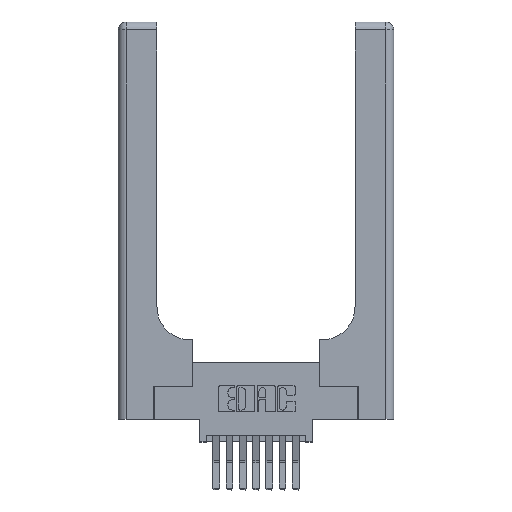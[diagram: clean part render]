
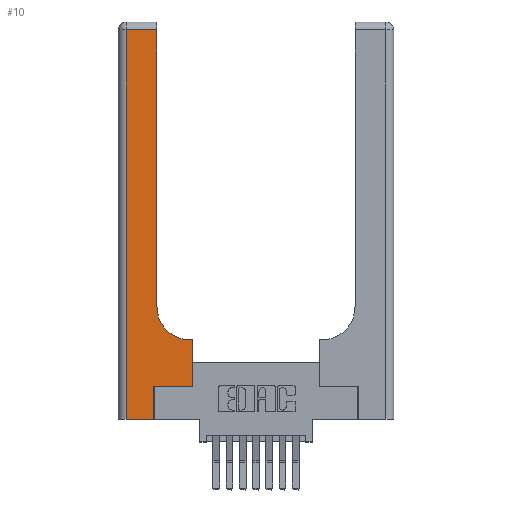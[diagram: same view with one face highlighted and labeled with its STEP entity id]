
A CAD part, top view. The second image highlights one B-rep face of the part: STEP entity #10.
In plain terms, the highlighted planar face has unit normal (0, 0, 1).
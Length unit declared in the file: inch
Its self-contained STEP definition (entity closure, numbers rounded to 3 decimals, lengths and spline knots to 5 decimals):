
#10 = ADVANCED_FACE ( 'NONE', ( #7738 ), #1130, .F. ) ;
#654 = LINE ( 'NONE', #7620, #6672 ) ;
#670 = CARTESIAN_POINT ( 'NONE',  ( 0.2915, 0.6, 0.37 ) ) ;
#739 = VECTOR ( 'NONE', #13479, 39.37008 ) ;
#786 = LINE ( 'NONE', #11193, #13255 ) ;
#826 = ORIENTED_EDGE ( 'NONE', *, *, #11435, .T. ) ;
#1130 = PLANE ( 'NONE',  #12716 ) ;
#1564 = ORIENTED_EDGE ( 'NONE', *, *, #3836, .T. ) ;
#1618 = LINE ( 'NONE', #4243, #4477 ) ;
#1707 = CARTESIAN_POINT ( 'NONE',  ( 0.5415, 0.85, 0.37 ) ) ;
#1835 = CARTESIAN_POINT ( 'NONE',  ( 0.06, 2.94, 0.37 ) ) ;
#2372 = ORIENTED_EDGE ( 'NONE', *, *, #14680, .T. ) ;
#2967 = DIRECTION ( 'NONE',  ( 1., 0., 0. ) ) ;
#3564 = VERTEX_POINT ( 'NONE', #5213 ) ;
#3594 = CARTESIAN_POINT ( 'NONE',  ( 0.2915, 3., 0.37 ) ) ;
#3836 = EDGE_CURVE ( 'NONE', #8129, #15580, #4797, .T. ) ;
#3838 = CARTESIAN_POINT ( 'NONE',  ( 0.06, 3., 0.37 ) ) ;
#4243 = CARTESIAN_POINT ( 'NONE',  ( 0.269, 0.25, 0.37 ) ) ;
#4425 = ORIENTED_EDGE ( 'NONE', *, *, #7631, .T. ) ;
#4477 = VECTOR ( 'NONE', #11522, 39.37008 ) ;
#4797 = LINE ( 'NONE', #6931, #7634 ) ;
#5213 = CARTESIAN_POINT ( 'NONE',  ( 0.2915, 2.94, 0.37 ) ) ;
#5412 = EDGE_CURVE ( 'NONE', #14479, #10782, #786, .T. ) ;
#5531 = VERTEX_POINT ( 'NONE', #1835 ) ;
#5629 = EDGE_LOOP ( 'NONE', ( #10140, #826, #4425, #10887, #1564, #14407, #8391, #11648, #2372 ) ) ;
#6672 = VECTOR ( 'NONE', #8851, 39.37008 ) ;
#6785 = EDGE_CURVE ( 'NONE', #8385, #3564, #14325, .T. ) ;
#6931 = CARTESIAN_POINT ( 'NONE',  ( 0.269, 0., 0.37 ) ) ;
#6965 = DIRECTION ( 'NONE',  ( 0., 0., -1. ) ) ;
#7145 = LINE ( 'NONE', #3838, #739 ) ;
#7150 = CARTESIAN_POINT ( 'NONE',  ( 0.06, 0., 0.37 ) ) ;
#7544 = DIRECTION ( 'NONE',  ( 0., 1., 0. ) ) ;
#7587 = VECTOR ( 'NONE', #14410, 39.37008 ) ;
#7620 = CARTESIAN_POINT ( 'NONE',  ( 0., 2.94, 0.37 ) ) ;
#7631 = EDGE_CURVE ( 'NONE', #5531, #14396, #7145, .T. ) ;
#7634 = VECTOR ( 'NONE', #11798, 39.37008 ) ;
#7738 = FACE_OUTER_BOUND ( 'NONE', #5629, .T. ) ;
#8129 = VERTEX_POINT ( 'NONE', #12398 ) ;
#8385 = VERTEX_POINT ( 'NONE', #11726 ) ;
#8391 = ORIENTED_EDGE ( 'NONE', *, *, #5412, .T. ) ;
#8716 = CIRCLE ( 'NONE', #13418, 0.25 ) ;
#8841 = DIRECTION ( 'NONE',  ( 0., 1., 0. ) ) ;
#8851 = DIRECTION ( 'NONE',  ( -1., 0., 0. ) ) ;
#9270 = VERTEX_POINT ( 'NONE', #13484 ) ;
#9622 = CARTESIAN_POINT ( 'NONE',  ( 0., 0., 0.37 ) ) ;
#10137 = EDGE_CURVE ( 'NONE', #15580, #14479, #1618, .T. ) ;
#10140 = ORIENTED_EDGE ( 'NONE', *, *, #6785, .T. ) ;
#10224 = DIRECTION ( 'NONE',  ( 0., 0., -1. ) ) ;
#10391 = DIRECTION ( 'NONE',  ( -1., 0., 0. ) ) ;
#10782 = VERTEX_POINT ( 'NONE', #11017 ) ;
#10857 = LINE ( 'NONE', #9622, #7587 ) ;
#10887 = ORIENTED_EDGE ( 'NONE', *, *, #13054, .T. ) ;
#11005 = DIRECTION ( 'NONE',  ( -1., 0., 0. ) ) ;
#11017 = CARTESIAN_POINT ( 'NONE',  ( 0.5585, 0.6, 0.37 ) ) ;
#11193 = CARTESIAN_POINT ( 'NONE',  ( 0.5585, 0.25, 0.37 ) ) ;
#11435 = EDGE_CURVE ( 'NONE', #3564, #5531, #654, .T. ) ;
#11522 = DIRECTION ( 'NONE',  ( 1., 0., 0. ) ) ;
#11648 = ORIENTED_EDGE ( 'NONE', *, *, #12719, .T. ) ;
#11726 = CARTESIAN_POINT ( 'NONE',  ( 0.2915, 0.85, 0.37 ) ) ;
#11798 = DIRECTION ( 'NONE',  ( 0., 1., 0. ) ) ;
#12170 = VECTOR ( 'NONE', #10391, 39.37008 ) ;
#12398 = CARTESIAN_POINT ( 'NONE',  ( 0.269, 0., 0.37 ) ) ;
#12716 = AXIS2_PLACEMENT_3D ( 'NONE', #14660, #6965, #11005 ) ;
#12719 = EDGE_CURVE ( 'NONE', #10782, #9270, #12910, .T. ) ;
#12910 = LINE ( 'NONE', #670, #12170 ) ;
#13054 = EDGE_CURVE ( 'NONE', #14396, #8129, #10857, .T. ) ;
#13255 = VECTOR ( 'NONE', #7544, 39.37008 ) ;
#13418 = AXIS2_PLACEMENT_3D ( 'NONE', #1707, #10224, #2967 ) ;
#13479 = DIRECTION ( 'NONE',  ( 0., -1., 0. ) ) ;
#13484 = CARTESIAN_POINT ( 'NONE',  ( 0.5415, 0.6, 0.37 ) ) ;
#14325 = LINE ( 'NONE', #3594, #15069 ) ;
#14390 = CARTESIAN_POINT ( 'NONE',  ( 0.269, 0.25, 0.37 ) ) ;
#14396 = VERTEX_POINT ( 'NONE', #7150 ) ;
#14407 = ORIENTED_EDGE ( 'NONE', *, *, #10137, .T. ) ;
#14410 = DIRECTION ( 'NONE',  ( 1., 0., 0. ) ) ;
#14479 = VERTEX_POINT ( 'NONE', #14534 ) ;
#14534 = CARTESIAN_POINT ( 'NONE',  ( 0.5585, 0.25, 0.37 ) ) ;
#14660 = CARTESIAN_POINT ( 'NONE',  ( 0., 3., 0.37 ) ) ;
#14680 = EDGE_CURVE ( 'NONE', #9270, #8385, #8716, .T. ) ;
#15069 = VECTOR ( 'NONE', #8841, 39.37008 ) ;
#15580 = VERTEX_POINT ( 'NONE', #14390 ) ;
